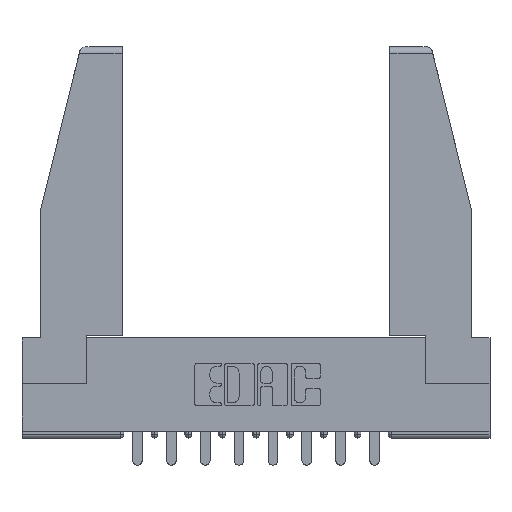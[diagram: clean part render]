
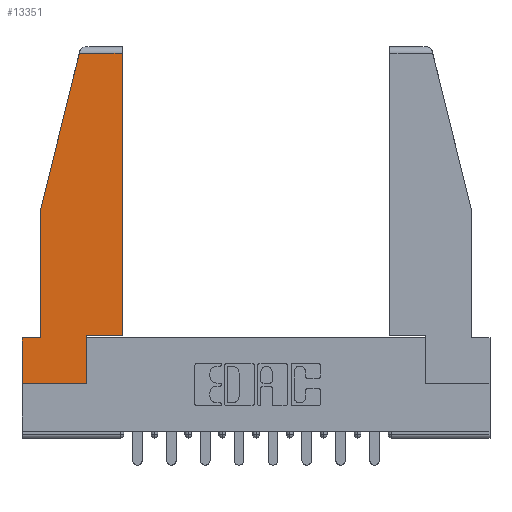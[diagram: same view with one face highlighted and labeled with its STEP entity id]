
A CAD part, top view. The second image highlights one B-rep face of the part: STEP entity #13351.
In plain terms, the highlighted planar face has unit normal (0, 0, 1).
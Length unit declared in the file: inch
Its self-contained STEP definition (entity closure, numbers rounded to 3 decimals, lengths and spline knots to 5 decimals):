
#297 = CARTESIAN_POINT ( 'NONE',  ( 0.086, 0.21, 0. ) ) ;
#319 = CARTESIAN_POINT ( 'NONE',  ( 0., 0.21, 0. ) ) ;
#365 = EDGE_CURVE ( 'NONE', #9007, #9385, #10823, .T. ) ;
#393 = CARTESIAN_POINT ( 'NONE',  ( 0.2636, 1.52, 0. ) ) ;
#620 = VECTOR ( 'NONE', #5478, 39.37008 ) ;
#994 = EDGE_CURVE ( 'NONE', #9385, #4759, #7852, .T. ) ;
#1186 = ORIENTED_EDGE ( 'NONE', *, *, #3766, .T. ) ;
#1558 = LINE ( 'NONE', #4622, #12179 ) ;
#1615 = LINE ( 'NONE', #2824, #13718 ) ;
#1724 = DIRECTION ( 'NONE',  ( 0., 1., 0. ) ) ;
#2168 = VECTOR ( 'NONE', #5298, 39.37008 ) ;
#2184 = CARTESIAN_POINT ( 'NONE',  ( 0.297, 0., 0. ) ) ;
#2241 = DIRECTION ( 'NONE',  ( 0., 0., 1. ) ) ;
#2374 = VECTOR ( 'NONE', #1724, 39.37008 ) ;
#2643 = CARTESIAN_POINT ( 'NONE',  ( 0.297, 0.223, 0. ) ) ;
#2742 = VERTEX_POINT ( 'NONE', #319 ) ;
#2824 = CARTESIAN_POINT ( 'NONE',  ( 0., 0.21, 0. ) ) ;
#2968 = CARTESIAN_POINT ( 'NONE',  ( 0.461, 0.223, 0. ) ) ;
#3014 = AXIS2_PLACEMENT_3D ( 'NONE', #6915, #2241, #12859 ) ;
#3348 = EDGE_CURVE ( 'NONE', #4782, #7244, #6716, .T. ) ;
#3408 = VECTOR ( 'NONE', #7958, 39.37008 ) ;
#3531 = ORIENTED_EDGE ( 'NONE', *, *, #10039, .T. ) ;
#3766 = EDGE_CURVE ( 'NONE', #7244, #7836, #12870, .T. ) ;
#3949 = DIRECTION ( 'NONE',  ( 0., 1., 0. ) ) ;
#4047 = ORIENTED_EDGE ( 'NONE', *, *, #994, .T. ) ;
#4537 = CARTESIAN_POINT ( 'NONE',  ( 0., 0.21, 0. ) ) ;
#4622 = CARTESIAN_POINT ( 'NONE',  ( 0.086, 0.8, 0. ) ) ;
#4759 = VERTEX_POINT ( 'NONE', #393 ) ;
#4782 = VERTEX_POINT ( 'NONE', #5081 ) ;
#5072 = DIRECTION ( 'NONE',  ( 0., -1., 0. ) ) ;
#5081 = CARTESIAN_POINT ( 'NONE',  ( 0., 0., 0. ) ) ;
#5298 = DIRECTION ( 'NONE',  ( -1., 0., 0. ) ) ;
#5478 = DIRECTION ( 'NONE',  ( -0.239, -0.971, 0. ) ) ;
#5721 = CARTESIAN_POINT ( 'NONE',  ( 0., 0., 0. ) ) ;
#5747 = VECTOR ( 'NONE', #12691, 39.37008 ) ;
#5752 = VERTEX_POINT ( 'NONE', #7595 ) ;
#6178 = EDGE_LOOP ( 'NONE', ( #14468, #4047, #8829, #14196, #10615, #3531, #9034, #1186, #12863 ) ) ;
#6716 = LINE ( 'NONE', #5721, #3408 ) ;
#6915 = CARTESIAN_POINT ( 'NONE',  ( 0., 0., 0. ) ) ;
#7039 = EDGE_CURVE ( 'NONE', #7836, #9007, #13885, .T. ) ;
#7081 = DIRECTION ( 'NONE',  ( 0., -1., 0. ) ) ;
#7244 = VERTEX_POINT ( 'NONE', #2184 ) ;
#7595 = CARTESIAN_POINT ( 'NONE',  ( 0.086, 0.8, 0. ) ) ;
#7836 = VERTEX_POINT ( 'NONE', #2643 ) ;
#7852 = LINE ( 'NONE', #11042, #2168 ) ;
#7958 = DIRECTION ( 'NONE',  ( 1., 0., 0. ) ) ;
#8118 = EDGE_CURVE ( 'NONE', #5752, #13438, #1558, .T. ) ;
#8715 = FACE_OUTER_BOUND ( 'NONE', #6178, .T. ) ;
#8829 = ORIENTED_EDGE ( 'NONE', *, *, #14972, .T. ) ;
#8858 = CARTESIAN_POINT ( 'NONE',  ( 0.461, 0.223, 0. ) ) ;
#9007 = VERTEX_POINT ( 'NONE', #2968 ) ;
#9034 = ORIENTED_EDGE ( 'NONE', *, *, #3348, .T. ) ;
#9385 = VERTEX_POINT ( 'NONE', #12736 ) ;
#9752 = VECTOR ( 'NONE', #3949, 39.37008 ) ;
#9844 = EDGE_CURVE ( 'NONE', #13438, #2742, #11406, .T. ) ;
#10039 = EDGE_CURVE ( 'NONE', #2742, #4782, #1615, .T. ) ;
#10142 = CARTESIAN_POINT ( 'NONE',  ( 0.297, 0.223, 0. ) ) ;
#10521 = LINE ( 'NONE', #14771, #620 ) ;
#10615 = ORIENTED_EDGE ( 'NONE', *, *, #9844, .T. ) ;
#10823 = LINE ( 'NONE', #8858, #2374 ) ;
#10981 = CARTESIAN_POINT ( 'NONE',  ( 0.297, 0., 0. ) ) ;
#11042 = CARTESIAN_POINT ( 'NONE',  ( 0., 1.52, 0. ) ) ;
#11157 = DIRECTION ( 'NONE',  ( 1., 0., 0. ) ) ;
#11406 = LINE ( 'NONE', #4537, #5747 ) ;
#12179 = VECTOR ( 'NONE', #7081, 39.37008 ) ;
#12691 = DIRECTION ( 'NONE',  ( -1., 0., 0. ) ) ;
#12736 = CARTESIAN_POINT ( 'NONE',  ( 0.461, 1.52, 0. ) ) ;
#12859 = DIRECTION ( 'NONE',  ( 1., 0., 0. ) ) ;
#12863 = ORIENTED_EDGE ( 'NONE', *, *, #7039, .T. ) ;
#12870 = LINE ( 'NONE', #10981, #9752 ) ;
#13351 = ADVANCED_FACE ( 'NONE', ( #8715 ), #13931, .T. ) ;
#13438 = VERTEX_POINT ( 'NONE', #297 ) ;
#13718 = VECTOR ( 'NONE', #5072, 39.37008 ) ;
#13885 = LINE ( 'NONE', #10142, #14421 ) ;
#13931 = PLANE ( 'NONE',  #3014 ) ;
#14196 = ORIENTED_EDGE ( 'NONE', *, *, #8118, .T. ) ;
#14421 = VECTOR ( 'NONE', #11157, 39.37008 ) ;
#14468 = ORIENTED_EDGE ( 'NONE', *, *, #365, .T. ) ;
#14771 = CARTESIAN_POINT ( 'NONE',  ( 0.271, 1.55, 0. ) ) ;
#14972 = EDGE_CURVE ( 'NONE', #4759, #5752, #10521, .T. ) ;
